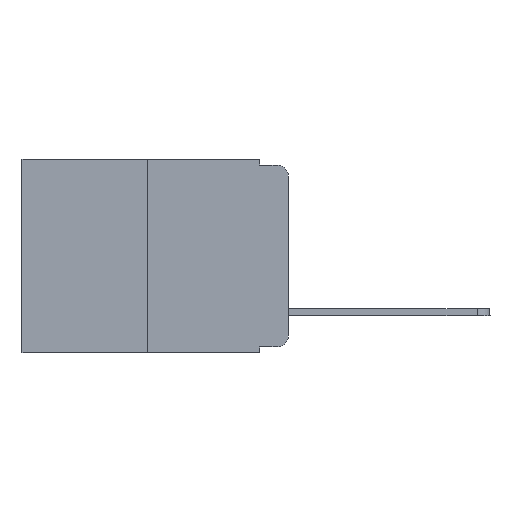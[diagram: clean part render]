
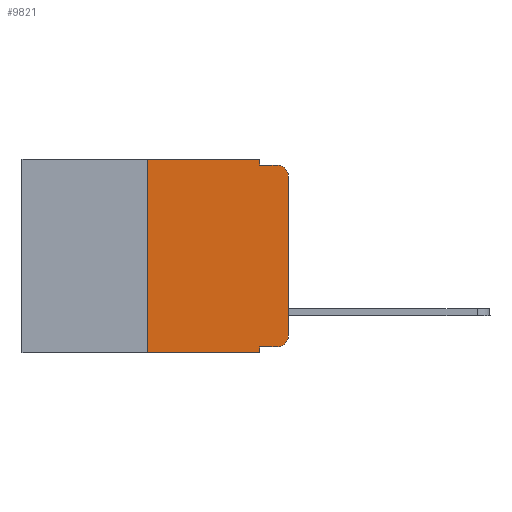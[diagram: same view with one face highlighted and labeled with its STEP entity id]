
A CAD part, left-side view. The second image highlights one B-rep face of the part: STEP entity #9821.
In plain terms, the highlighted planar face has unit normal (-1, 0, 0).
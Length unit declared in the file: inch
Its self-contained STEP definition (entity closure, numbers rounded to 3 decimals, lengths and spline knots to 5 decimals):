
#83 = CARTESIAN_POINT ( 'NONE',  ( 0., 0.051, -0.01 ) ) ;
#258 = VERTEX_POINT ( 'NONE', #6139 ) ;
#593 = CARTESIAN_POINT ( 'NONE',  ( 0., 0.051, 0. ) ) ;
#810 = LINE ( 'NONE', #1626, #9650 ) ;
#843 = EDGE_CURVE ( 'NONE', #9551, #1493, #810, .T. ) ;
#1017 = ORIENTED_EDGE ( 'NONE', *, *, #3793, .T. ) ;
#1102 = CARTESIAN_POINT ( 'NONE',  ( 0., 0., -0.03 ) ) ;
#1239 = CARTESIAN_POINT ( 'NONE',  ( 0., 0.02, -0.313 ) ) ;
#1297 = CIRCLE ( 'NONE', #8391, 0.02 ) ;
#1301 = DIRECTION ( 'NONE',  ( 0., 0., -1. ) ) ;
#1338 = CARTESIAN_POINT ( 'NONE',  ( 0., 0.051, -0.333 ) ) ;
#1493 = VERTEX_POINT ( 'NONE', #4213 ) ;
#1626 = CARTESIAN_POINT ( 'NONE',  ( 0., 0.25, 0. ) ) ;
#1804 = CARTESIAN_POINT ( 'NONE',  ( 0., 0.473, 0. ) ) ;
#1992 = LINE ( 'NONE', #1338, #4779 ) ;
#2100 = CARTESIAN_POINT ( 'NONE',  ( 0., 0.051, 0. ) ) ;
#2152 = DIRECTION ( 'NONE',  ( 0., -1., 0. ) ) ;
#2163 = DIRECTION ( 'NONE',  ( -1., 0., 0. ) ) ;
#2781 = EDGE_CURVE ( 'NONE', #1493, #7589, #5641, .T. ) ;
#2917 = CARTESIAN_POINT ( 'NONE',  ( 0., 0.02, -0.01 ) ) ;
#2950 = EDGE_CURVE ( 'NONE', #258, #9155, #1992, .T. ) ;
#2998 = CARTESIAN_POINT ( 'NONE',  ( 0., 0.02, -0.03 ) ) ;
#3069 = CARTESIAN_POINT ( 'NONE',  ( 0., 0., -0.313 ) ) ;
#3169 = LINE ( 'NONE', #593, #4010 ) ;
#3338 = AXIS2_PLACEMENT_3D ( 'NONE', #7043, #10615, #5444 ) ;
#3643 = DIRECTION ( 'NONE',  ( 0., 0., 1. ) ) ;
#3716 = VECTOR ( 'NONE', #5697, 39.37008 ) ;
#3793 = EDGE_CURVE ( 'NONE', #11474, #6880, #11266, .T. ) ;
#3863 = ORIENTED_EDGE ( 'NONE', *, *, #2781, .F. ) ;
#3877 = EDGE_CURVE ( 'NONE', #9155, #5676, #1297, .T. ) ;
#3892 = DIRECTION ( 'NONE',  ( -1., 0., 0. ) ) ;
#4010 = VECTOR ( 'NONE', #1301, 39.37008 ) ;
#4213 = CARTESIAN_POINT ( 'NONE',  ( 0., 0.25, 0. ) ) ;
#4519 = VECTOR ( 'NONE', #8169, 39.37008 ) ;
#4705 = LINE ( 'NONE', #10749, #6785 ) ;
#4779 = VECTOR ( 'NONE', #2152, 39.37008 ) ;
#4827 = DIRECTION ( 'NONE',  ( 0., 0., -1. ) ) ;
#4990 = LINE ( 'NONE', #2100, #3716 ) ;
#5092 = DIRECTION ( 'NONE',  ( 0., -1., 0. ) ) ;
#5242 = CARTESIAN_POINT ( 'NONE',  ( 0., 0.051, -0.01 ) ) ;
#5409 = ORIENTED_EDGE ( 'NONE', *, *, #2950, .T. ) ;
#5444 = DIRECTION ( 'NONE',  ( 0., 0., -1. ) ) ;
#5498 = VERTEX_POINT ( 'NONE', #5242 ) ;
#5641 = LINE ( 'NONE', #1804, #4519 ) ;
#5676 = VERTEX_POINT ( 'NONE', #3069 ) ;
#5697 = DIRECTION ( 'NONE',  ( 0., 0., -1. ) ) ;
#6139 = CARTESIAN_POINT ( 'NONE',  ( 0., 0.051, -0.333 ) ) ;
#6277 = ORIENTED_EDGE ( 'NONE', *, *, #10135, .F. ) ;
#6505 = FACE_OUTER_BOUND ( 'NONE', #9228, .T. ) ;
#6668 = EDGE_CURVE ( 'NONE', #5498, #6880, #11115, .T. ) ;
#6785 = VECTOR ( 'NONE', #3643, 39.37008 ) ;
#6880 = VERTEX_POINT ( 'NONE', #2917 ) ;
#7007 = ORIENTED_EDGE ( 'NONE', *, *, #9532, .F. ) ;
#7043 = CARTESIAN_POINT ( 'NONE',  ( 0., 0.473, 0. ) ) ;
#7310 = DIRECTION ( 'NONE',  ( 0., 0., -1. ) ) ;
#7497 = CARTESIAN_POINT ( 'NONE',  ( 0., 0.25, -0.343 ) ) ;
#7509 = ORIENTED_EDGE ( 'NONE', *, *, #9329, .T. ) ;
#7589 = VERTEX_POINT ( 'NONE', #8820 ) ;
#7711 = ORIENTED_EDGE ( 'NONE', *, *, #843, .F. ) ;
#7778 = ORIENTED_EDGE ( 'NONE', *, *, #6668, .F. ) ;
#7780 = CARTESIAN_POINT ( 'NONE',  ( 0., 0.051, -0.343 ) ) ;
#7894 = EDGE_CURVE ( 'NONE', #9551, #9031, #8033, .T. ) ;
#7989 = DIRECTION ( 'NONE',  ( 0., -1., 0. ) ) ;
#8033 = LINE ( 'NONE', #9599, #8716 ) ;
#8169 = DIRECTION ( 'NONE',  ( 0., -1., 0. ) ) ;
#8319 = AXIS2_PLACEMENT_3D ( 'NONE', #2998, #3892, #4827 ) ;
#8391 = AXIS2_PLACEMENT_3D ( 'NONE', #1239, #2163, #7310 ) ;
#8716 = VECTOR ( 'NONE', #5092, 39.37008 ) ;
#8746 = VECTOR ( 'NONE', #7989, 39.37008 ) ;
#8820 = CARTESIAN_POINT ( 'NONE',  ( 0., 0.051, 0. ) ) ;
#9031 = VERTEX_POINT ( 'NONE', #7780 ) ;
#9155 = VERTEX_POINT ( 'NONE', #9649 ) ;
#9228 = EDGE_LOOP ( 'NONE', ( #7509, #1017, #7778, #6277, #3863, #7711, #11279, #7007, #5409, #11139 ) ) ;
#9329 = EDGE_CURVE ( 'NONE', #5676, #11474, #4705, .T. ) ;
#9532 = EDGE_CURVE ( 'NONE', #258, #9031, #3169, .T. ) ;
#9551 = VERTEX_POINT ( 'NONE', #7497 ) ;
#9599 = CARTESIAN_POINT ( 'NONE',  ( 0., 0.473, -0.343 ) ) ;
#9649 = CARTESIAN_POINT ( 'NONE',  ( 0., 0.02, -0.333 ) ) ;
#9650 = VECTOR ( 'NONE', #11374, 39.37008 ) ;
#9676 = PLANE ( 'NONE',  #3338 ) ;
#9821 = ADVANCED_FACE ( 'NONE', ( #6505 ), #9676, .F. ) ;
#10135 = EDGE_CURVE ( 'NONE', #7589, #5498, #4990, .T. ) ;
#10615 = DIRECTION ( 'NONE',  ( 1., 0., 0. ) ) ;
#10749 = CARTESIAN_POINT ( 'NONE',  ( 0., 0., 0. ) ) ;
#11115 = LINE ( 'NONE', #83, #8746 ) ;
#11139 = ORIENTED_EDGE ( 'NONE', *, *, #3877, .T. ) ;
#11266 = CIRCLE ( 'NONE', #8319, 0.02 ) ;
#11279 = ORIENTED_EDGE ( 'NONE', *, *, #7894, .T. ) ;
#11374 = DIRECTION ( 'NONE',  ( 0., 0., 1. ) ) ;
#11474 = VERTEX_POINT ( 'NONE', #1102 ) ;
